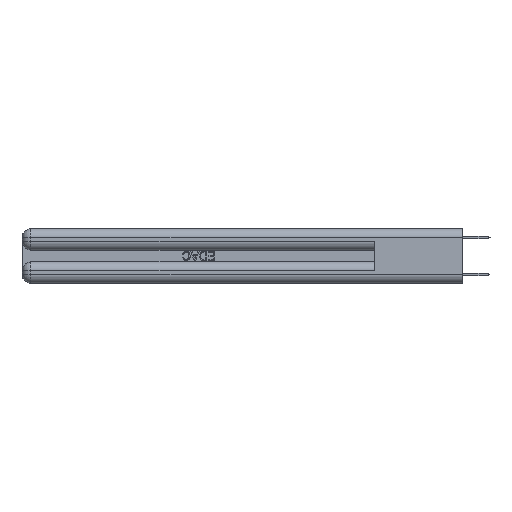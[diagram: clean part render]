
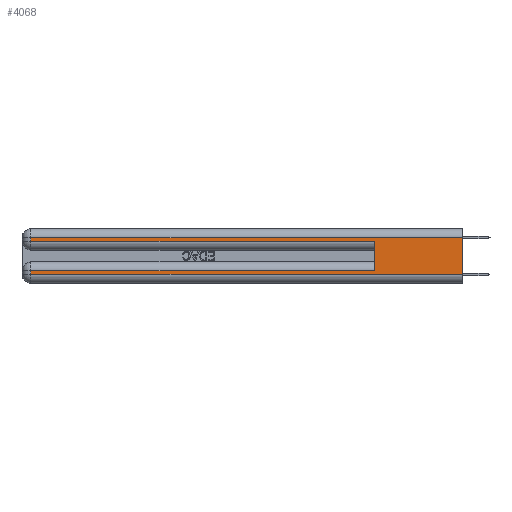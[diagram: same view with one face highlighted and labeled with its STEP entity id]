
A CAD part, left-side view. The second image highlights one B-rep face of the part: STEP entity #4068.
In plain terms, the highlighted planar face has unit normal (-1, 0, 0).
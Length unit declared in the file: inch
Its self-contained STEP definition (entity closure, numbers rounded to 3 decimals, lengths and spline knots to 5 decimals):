
#56 = VERTEX_POINT ( 'NONE', #4875 ) ;
#361 = DIRECTION ( 'NONE',  ( 0., -1., 0. ) ) ;
#443 = FACE_OUTER_BOUND ( 'NONE', #6065, .T. ) ;
#725 = LINE ( 'NONE', #9774, #27710 ) ;
#2023 = CARTESIAN_POINT ( 'NONE',  ( 0., 0.6, 0.145 ) ) ;
#2030 = CARTESIAN_POINT ( 'NONE',  ( 0., 0., 0.06 ) ) ;
#2076 = CARTESIAN_POINT ( 'NONE',  ( 0., 2.94, 0.37 ) ) ;
#2454 = LINE ( 'NONE', #11930, #14248 ) ;
#3722 = CARTESIAN_POINT ( 'NONE',  ( 0., 0., 0.085 ) ) ;
#4068 = ADVANCED_FACE ( 'NONE', ( #443 ), #20061, .F. ) ;
#4207 = ORIENTED_EDGE ( 'NONE', *, *, #27385, .F. ) ;
#4875 = CARTESIAN_POINT ( 'NONE',  ( 0., 2.94, 0.31 ) ) ;
#5067 = VECTOR ( 'NONE', #29347, 39.37008 ) ;
#5208 = CARTESIAN_POINT ( 'NONE',  ( 0., 0., 0.31 ) ) ;
#5670 = EDGE_CURVE ( 'NONE', #26477, #28533, #12600, .T. ) ;
#5802 = LINE ( 'NONE', #29441, #5067 ) ;
#6065 = EDGE_LOOP ( 'NONE', ( #17757, #11400, #12563, #15079, #4207, #19779, #16405, #14498 ) ) ;
#6863 = CARTESIAN_POINT ( 'NONE',  ( 0., 2.94, 0.37 ) ) ;
#6961 = CARTESIAN_POINT ( 'NONE',  ( 0., 2.94, 0.085 ) ) ;
#7046 = EDGE_CURVE ( 'NONE', #21378, #21956, #725, .T. ) ;
#7998 = CARTESIAN_POINT ( 'NONE',  ( 0., 0.6, 0.285 ) ) ;
#8668 = LINE ( 'NONE', #3722, #25274 ) ;
#8990 = CARTESIAN_POINT ( 'NONE',  ( 0., 2.94, 0.285 ) ) ;
#9774 = CARTESIAN_POINT ( 'NONE',  ( 0., 0., 0.285 ) ) ;
#9961 = EDGE_CURVE ( 'NONE', #28533, #13079, #2454, .T. ) ;
#10712 = EDGE_CURVE ( 'NONE', #12055, #56, #20800, .T. ) ;
#10968 = EDGE_CURVE ( 'NONE', #28868, #26477, #8668, .T. ) ;
#11230 = VECTOR ( 'NONE', #21858, 39.37008 ) ;
#11400 = ORIENTED_EDGE ( 'NONE', *, *, #10712, .T. ) ;
#11580 = DIRECTION ( 'NONE',  ( 0., 0., -1. ) ) ;
#11930 = CARTESIAN_POINT ( 'NONE',  ( 0., 0., 0.06 ) ) ;
#12055 = VERTEX_POINT ( 'NONE', #5208 ) ;
#12408 = VECTOR ( 'NONE', #23693, 39.37008 ) ;
#12563 = ORIENTED_EDGE ( 'NONE', *, *, #23754, .T. ) ;
#12600 = LINE ( 'NONE', #2076, #18490 ) ;
#13079 = VERTEX_POINT ( 'NONE', #2030 ) ;
#13590 = VECTOR ( 'NONE', #23364, 39.37008 ) ;
#14248 = VECTOR ( 'NONE', #16356, 39.37008 ) ;
#14498 = ORIENTED_EDGE ( 'NONE', *, *, #9961, .T. ) ;
#15079 = ORIENTED_EDGE ( 'NONE', *, *, #7046, .T. ) ;
#15760 = DIRECTION ( 'NONE',  ( 0., 1., 0. ) ) ;
#16356 = DIRECTION ( 'NONE',  ( 0., -1., 0. ) ) ;
#16405 = ORIENTED_EDGE ( 'NONE', *, *, #5670, .T. ) ;
#17757 = ORIENTED_EDGE ( 'NONE', *, *, #28181, .F. ) ;
#18490 = VECTOR ( 'NONE', #11580, 39.37008 ) ;
#18654 = LINE ( 'NONE', #6863, #12408 ) ;
#19779 = ORIENTED_EDGE ( 'NONE', *, *, #10968, .T. ) ;
#20061 = PLANE ( 'NONE',  #29761 ) ;
#20622 = CARTESIAN_POINT ( 'NONE',  ( 0., 0.6, 0.085 ) ) ;
#20800 = LINE ( 'NONE', #24267, #11230 ) ;
#21378 = VERTEX_POINT ( 'NONE', #8990 ) ;
#21858 = DIRECTION ( 'NONE',  ( 0., 1., 0. ) ) ;
#21956 = VERTEX_POINT ( 'NONE', #7998 ) ;
#23364 = DIRECTION ( 'NONE',  ( 0., 0., 1. ) ) ;
#23693 = DIRECTION ( 'NONE',  ( 0., 0., -1. ) ) ;
#23754 = EDGE_CURVE ( 'NONE', #56, #21378, #18654, .T. ) ;
#23761 = CARTESIAN_POINT ( 'NONE',  ( 0., 2.94, 0.06 ) ) ;
#24267 = CARTESIAN_POINT ( 'NONE',  ( 0., 0., 0.31 ) ) ;
#24850 = CARTESIAN_POINT ( 'NONE',  ( 0., 0., 0.37 ) ) ;
#25274 = VECTOR ( 'NONE', #15760, 39.37008 ) ;
#26187 = LINE ( 'NONE', #2023, #13590 ) ;
#26477 = VERTEX_POINT ( 'NONE', #6961 ) ;
#27385 = EDGE_CURVE ( 'NONE', #28868, #21956, #26187, .T. ) ;
#27710 = VECTOR ( 'NONE', #361, 39.37008 ) ;
#28181 = EDGE_CURVE ( 'NONE', #12055, #13079, #5802, .T. ) ;
#28533 = VERTEX_POINT ( 'NONE', #23761 ) ;
#28868 = VERTEX_POINT ( 'NONE', #20622 ) ;
#29347 = DIRECTION ( 'NONE',  ( 0., 0., -1. ) ) ;
#29441 = CARTESIAN_POINT ( 'NONE',  ( 0., 0., 0.37 ) ) ;
#29761 = AXIS2_PLACEMENT_3D ( 'NONE', #24850, #29956, #29857 ) ;
#29857 = DIRECTION ( 'NONE',  ( 0., 0., -1. ) ) ;
#29956 = DIRECTION ( 'NONE',  ( 1., 0., 0. ) ) ;
